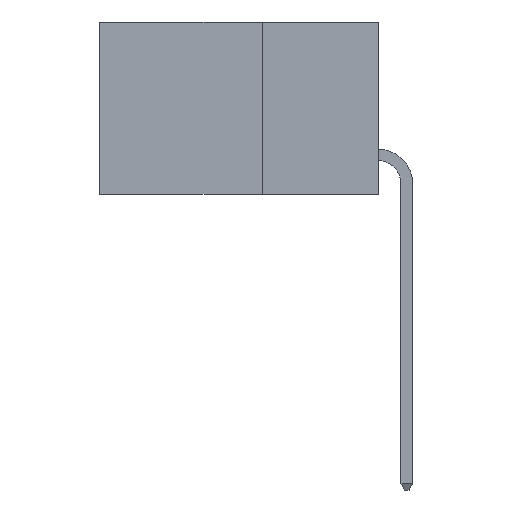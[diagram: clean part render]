
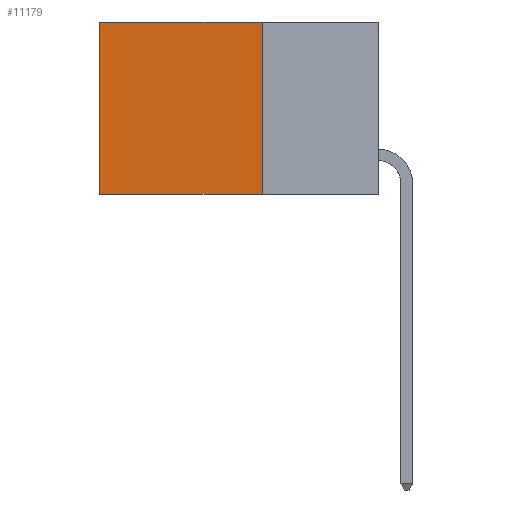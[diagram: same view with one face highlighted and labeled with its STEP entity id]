
A CAD part, left-side view. The second image highlights one B-rep face of the part: STEP entity #11179.
In plain terms, the highlighted planar face has unit normal (-1, 0, 0).
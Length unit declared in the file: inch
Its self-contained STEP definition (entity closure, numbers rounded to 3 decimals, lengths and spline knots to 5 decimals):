
#135 = DIRECTION ( 'NONE',  ( 1., 0., 0. ) ) ;
#379 = FACE_OUTER_BOUND ( 'NONE', #15115, .T. ) ;
#1306 = CARTESIAN_POINT ( 'NONE',  ( 0.2615, 0.25, -0.37 ) ) ;
#1800 = CARTESIAN_POINT ( 'NONE',  ( 0.2615, 0.25, 0. ) ) ;
#2503 = ORIENTED_EDGE ( 'NONE', *, *, #14426, .F. ) ;
#2891 = VECTOR ( 'NONE', #4260, 39.37008 ) ;
#3022 = DIRECTION ( 'NONE',  ( 0., 1., 0. ) ) ;
#3071 = CARTESIAN_POINT ( 'NONE',  ( 0.2615, 0.25, -0.37 ) ) ;
#3235 = VERTEX_POINT ( 'NONE', #4779 ) ;
#4007 = LINE ( 'NONE', #1800, #12570 ) ;
#4260 = DIRECTION ( 'NONE',  ( 0., 1., 0. ) ) ;
#4552 = EDGE_CURVE ( 'NONE', #6967, #6149, #13035, .T. ) ;
#4779 = CARTESIAN_POINT ( 'NONE',  ( 0.2615, 0.25, -0.37 ) ) ;
#5289 = VERTEX_POINT ( 'NONE', #12425 ) ;
#5543 = LINE ( 'NONE', #7217, #8297 ) ;
#5944 = VECTOR ( 'NONE', #12241, 39.37008 ) ;
#6075 = PLANE ( 'NONE',  #8264 ) ;
#6080 = CARTESIAN_POINT ( 'NONE',  ( 0.2615, 0.6, 0. ) ) ;
#6149 = VERTEX_POINT ( 'NONE', #10508 ) ;
#6967 = VERTEX_POINT ( 'NONE', #6080 ) ;
#7217 = CARTESIAN_POINT ( 'NONE',  ( 0.2615, 0.25, -0.37 ) ) ;
#7380 = ORIENTED_EDGE ( 'NONE', *, *, #4552, .T. ) ;
#7752 = ORIENTED_EDGE ( 'NONE', *, *, #12563, .F. ) ;
#8264 = AXIS2_PLACEMENT_3D ( 'NONE', #1306, #135, #8436 ) ;
#8297 = VECTOR ( 'NONE', #8398, 39.37008 ) ;
#8398 = DIRECTION ( 'NONE',  ( 0., 0., -1. ) ) ;
#8436 = DIRECTION ( 'NONE',  ( 0., 0., -1. ) ) ;
#8756 = CARTESIAN_POINT ( 'NONE',  ( 0.2615, 0.6, -0.37 ) ) ;
#9083 = ORIENTED_EDGE ( 'NONE', *, *, #14397, .T. ) ;
#10508 = CARTESIAN_POINT ( 'NONE',  ( 0.2615, 0.6, -0.37 ) ) ;
#11179 = ADVANCED_FACE ( 'NONE', ( #379 ), #6075, .F. ) ;
#12209 = LINE ( 'NONE', #3071, #2891 ) ;
#12241 = DIRECTION ( 'NONE',  ( 0., 0., -1. ) ) ;
#12425 = CARTESIAN_POINT ( 'NONE',  ( 0.2615, 0.25, 0. ) ) ;
#12563 = EDGE_CURVE ( 'NONE', #5289, #3235, #5543, .T. ) ;
#12570 = VECTOR ( 'NONE', #3022, 39.37008 ) ;
#13035 = LINE ( 'NONE', #8756, #5944 ) ;
#14397 = EDGE_CURVE ( 'NONE', #5289, #6967, #4007, .T. ) ;
#14426 = EDGE_CURVE ( 'NONE', #3235, #6149, #12209, .T. ) ;
#15115 = EDGE_LOOP ( 'NONE', ( #7380, #2503, #7752, #9083 ) ) ;
